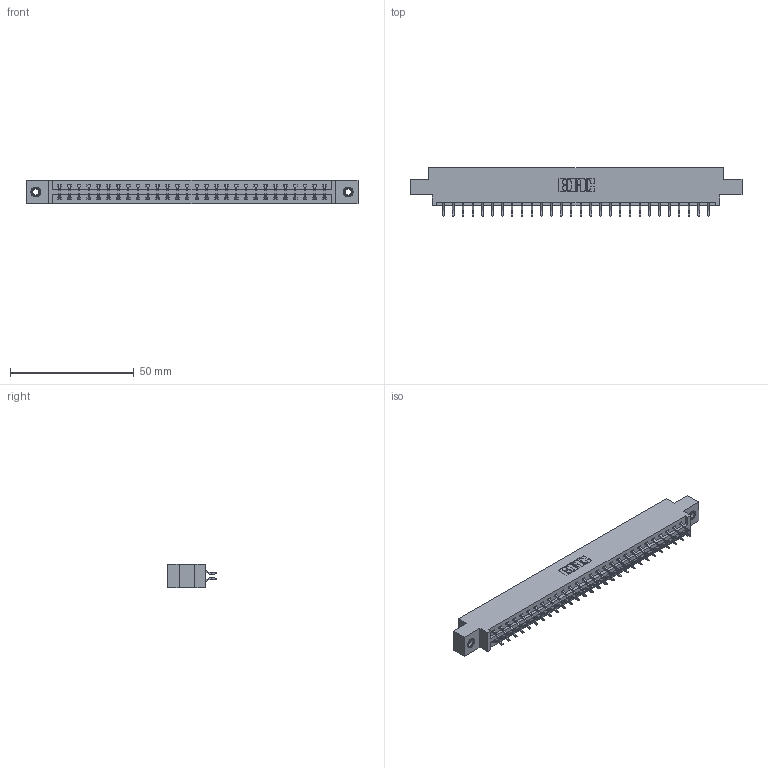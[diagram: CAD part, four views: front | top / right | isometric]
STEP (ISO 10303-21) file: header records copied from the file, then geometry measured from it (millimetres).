
FILE_DESCRIPTION (( 'STEP AP203' ), '1' );
FILE_NAME ('387-056-556-807.STEP', '2018-09-21T00:23:59', ( '' ), ( '' ), 'SwSTEP 2.0', 'SolidWorks 2016', '' );
FILE_SCHEMA (( 'CONFIG_CONTROL_DESIGN' ));
Length unit declared in the file: inch
Products named in the file (4): 387-056-556-807; 337 Part_0.170 Offset - 0.156 Dia-TI; 345-292-001_556 Tail; 345-250-001_345-250-005-103
Assembly tree (59 placements, depth 2):
  387-056-556-807
    337 Part_0.170 Offset - 0.156 Dia-TI
    345-292-001_556 Tail  x56
    345-250-001_345-250-005-103  x2
Bounding box: 133.96 x 19.57 x 9.4 mm (x, y, z)
Volume: 13798.1 mm3; surface area: 15547.5 mm2
Topology: 59 solids, 59 shells, 3538 faces, 10483 edges, 6906 vertices
Faces by surface type: plane 2458, cylinder 1064, cone 12, torus 4
Entity records: 25058 total; most frequent: CARTESIAN_POINT 4229, ORIENTED_EDGE 4146, DIRECTION 3643, EDGE_CURVE 2073, VECTOR 1917, LINE 1917, VERTEX_POINT 1376, AXIS2_PLACEMENT_3D 863
